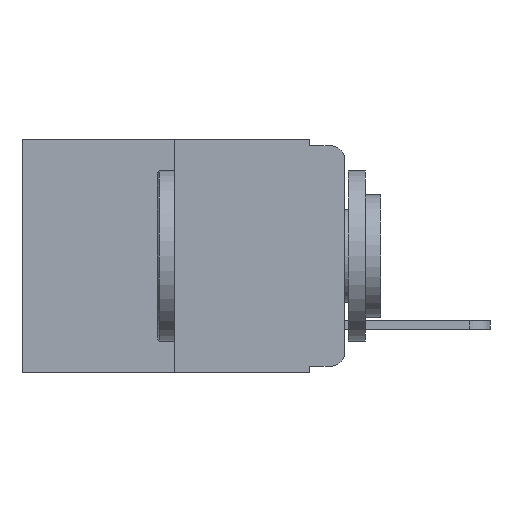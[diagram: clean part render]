
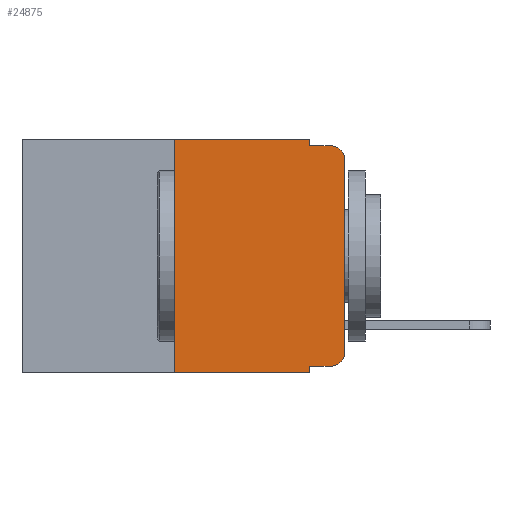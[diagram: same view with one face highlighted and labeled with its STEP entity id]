
A CAD part, left-side view. The second image highlights one B-rep face of the part: STEP entity #24875.
In plain terms, the highlighted planar face has unit normal (-1, 0, 0).
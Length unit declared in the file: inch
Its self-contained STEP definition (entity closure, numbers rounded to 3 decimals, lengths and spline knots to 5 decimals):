
#71 = CARTESIAN_POINT ( 'NONE',  ( 0., 0.02, -0.313 ) ) ;
#639 = LINE ( 'NONE', #1756, #17734 ) ;
#1099 = DIRECTION ( 'NONE',  ( 0., -1., 0. ) ) ;
#1131 = CARTESIAN_POINT ( 'NONE',  ( 0., 0.25, -0.343 ) ) ;
#1546 = CARTESIAN_POINT ( 'NONE',  ( 0., 0.02, -0.03 ) ) ;
#1626 = CARTESIAN_POINT ( 'NONE',  ( 0., 0.02, -0.01 ) ) ;
#1635 = VECTOR ( 'NONE', #22173, 39.37008 ) ;
#1756 = CARTESIAN_POINT ( 'NONE',  ( 0., 0.051, 0. ) ) ;
#1786 = DIRECTION ( 'NONE',  ( 1., 0., 0. ) ) ;
#1897 = VERTEX_POINT ( 'NONE', #18609 ) ;
#2009 = VECTOR ( 'NONE', #25522, 39.37008 ) ;
#2218 = DIRECTION ( 'NONE',  ( 0., 0., -1. ) ) ;
#2657 = LINE ( 'NONE', #11187, #24085 ) ;
#2782 = LINE ( 'NONE', #3222, #8509 ) ;
#2985 = EDGE_CURVE ( 'NONE', #10578, #13261, #21106, .T. ) ;
#3222 = CARTESIAN_POINT ( 'NONE',  ( 0., 0.25, 0. ) ) ;
#3359 = CARTESIAN_POINT ( 'NONE',  ( 0., 0.051, -0.333 ) ) ;
#3525 = EDGE_CURVE ( 'NONE', #11620, #23962, #18372, .T. ) ;
#3951 = LINE ( 'NONE', #20509, #20127 ) ;
#4475 = DIRECTION ( 'NONE',  ( 0., -1., 0. ) ) ;
#4498 = AXIS2_PLACEMENT_3D ( 'NONE', #71, #14825, #2218 ) ;
#4586 = ORIENTED_EDGE ( 'NONE', *, *, #13445, .F. ) ;
#4925 = CARTESIAN_POINT ( 'NONE',  ( 0., 0.051, -0.01 ) ) ;
#4945 = ORIENTED_EDGE ( 'NONE', *, *, #3525, .T. ) ;
#5041 = VECTOR ( 'NONE', #1099, 39.37008 ) ;
#5185 = ORIENTED_EDGE ( 'NONE', *, *, #8743, .T. ) ;
#5367 = CARTESIAN_POINT ( 'NONE',  ( 0., 0.473, -0.343 ) ) ;
#5506 = EDGE_CURVE ( 'NONE', #16760, #10805, #23183, .T. ) ;
#6530 = ORIENTED_EDGE ( 'NONE', *, *, #5506, .F. ) ;
#8509 = VECTOR ( 'NONE', #19526, 39.37008 ) ;
#8637 = DIRECTION ( 'NONE',  ( 0., 0., -1. ) ) ;
#8743 = EDGE_CURVE ( 'NONE', #22184, #13261, #20902, .T. ) ;
#9918 = CARTESIAN_POINT ( 'NONE',  ( 0., 0.051, 0. ) ) ;
#9970 = CARTESIAN_POINT ( 'NONE',  ( 0., 0.25, 0. ) ) ;
#10386 = EDGE_CURVE ( 'NONE', #14656, #16563, #22970, .T. ) ;
#10535 = ORIENTED_EDGE ( 'NONE', *, *, #12920, .T. ) ;
#10578 = VERTEX_POINT ( 'NONE', #24827 ) ;
#10805 = VERTEX_POINT ( 'NONE', #9918 ) ;
#11059 = DIRECTION ( 'NONE',  ( 0., 0., 1. ) ) ;
#11187 = CARTESIAN_POINT ( 'NONE',  ( 0., 0., 0. ) ) ;
#11620 = VERTEX_POINT ( 'NONE', #3359 ) ;
#12127 = CARTESIAN_POINT ( 'NONE',  ( 0., 0., -0.03 ) ) ;
#12531 = ORIENTED_EDGE ( 'NONE', *, *, #21675, .T. ) ;
#12798 = DIRECTION ( 'NONE',  ( 0., 0., -1. ) ) ;
#12803 = ORIENTED_EDGE ( 'NONE', *, *, #18561, .F. ) ;
#12889 = DIRECTION ( 'NONE',  ( -1., 0., 0. ) ) ;
#12920 = EDGE_CURVE ( 'NONE', #1897, #22184, #2657, .T. ) ;
#13261 = VERTEX_POINT ( 'NONE', #1626 ) ;
#13438 = ORIENTED_EDGE ( 'NONE', *, *, #2985, .F. ) ;
#13445 = EDGE_CURVE ( 'NONE', #11620, #16563, #639, .T. ) ;
#14656 = VERTEX_POINT ( 'NONE', #1131 ) ;
#14825 = DIRECTION ( 'NONE',  ( -1., 0., 0. ) ) ;
#15329 = ORIENTED_EDGE ( 'NONE', *, *, #10386, .T. ) ;
#16248 = PLANE ( 'NONE',  #16893 ) ;
#16304 = DIRECTION ( 'NONE',  ( 0., 0., -1. ) ) ;
#16328 = DIRECTION ( 'NONE',  ( 0., 0., -1. ) ) ;
#16563 = VERTEX_POINT ( 'NONE', #24960 ) ;
#16760 = VERTEX_POINT ( 'NONE', #9970 ) ;
#16893 = AXIS2_PLACEMENT_3D ( 'NONE', #22066, #1786, #16328 ) ;
#17421 = CIRCLE ( 'NONE', #4498, 0.02 ) ;
#17734 = VECTOR ( 'NONE', #16304, 39.37008 ) ;
#18372 = LINE ( 'NONE', #26027, #2009 ) ;
#18561 = EDGE_CURVE ( 'NONE', #14656, #16760, #2782, .T. ) ;
#18609 = CARTESIAN_POINT ( 'NONE',  ( 0., 0., -0.313 ) ) ;
#19124 = ORIENTED_EDGE ( 'NONE', *, *, #25003, .F. ) ;
#19276 = AXIS2_PLACEMENT_3D ( 'NONE', #1546, #12889, #12798 ) ;
#19526 = DIRECTION ( 'NONE',  ( 0., 0., 1. ) ) ;
#20127 = VECTOR ( 'NONE', #8637, 39.37008 ) ;
#20317 = EDGE_LOOP ( 'NONE', ( #10535, #5185, #13438, #19124, #6530, #12803, #15329, #4586, #4945, #12531 ) ) ;
#20509 = CARTESIAN_POINT ( 'NONE',  ( 0., 0.051, 0. ) ) ;
#20902 = CIRCLE ( 'NONE', #19276, 0.02 ) ;
#20972 = CARTESIAN_POINT ( 'NONE',  ( 0., 0.02, -0.333 ) ) ;
#21106 = LINE ( 'NONE', #4925, #5041 ) ;
#21675 = EDGE_CURVE ( 'NONE', #23962, #1897, #17421, .T. ) ;
#21772 = VECTOR ( 'NONE', #4475, 39.37008 ) ;
#22066 = CARTESIAN_POINT ( 'NONE',  ( 0., 0.473, 0. ) ) ;
#22173 = DIRECTION ( 'NONE',  ( 0., -1., 0. ) ) ;
#22184 = VERTEX_POINT ( 'NONE', #12127 ) ;
#22317 = CARTESIAN_POINT ( 'NONE',  ( 0., 0.473, 0. ) ) ;
#22566 = FACE_OUTER_BOUND ( 'NONE', #20317, .T. ) ;
#22970 = LINE ( 'NONE', #5367, #21772 ) ;
#23183 = LINE ( 'NONE', #22317, #1635 ) ;
#23962 = VERTEX_POINT ( 'NONE', #20972 ) ;
#24085 = VECTOR ( 'NONE', #11059, 39.37008 ) ;
#24827 = CARTESIAN_POINT ( 'NONE',  ( 0., 0.051, -0.01 ) ) ;
#24875 = ADVANCED_FACE ( 'NONE', ( #22566 ), #16248, .F. ) ;
#24960 = CARTESIAN_POINT ( 'NONE',  ( 0., 0.051, -0.343 ) ) ;
#25003 = EDGE_CURVE ( 'NONE', #10805, #10578, #3951, .T. ) ;
#25522 = DIRECTION ( 'NONE',  ( 0., -1., 0. ) ) ;
#26027 = CARTESIAN_POINT ( 'NONE',  ( 0., 0.051, -0.333 ) ) ;
